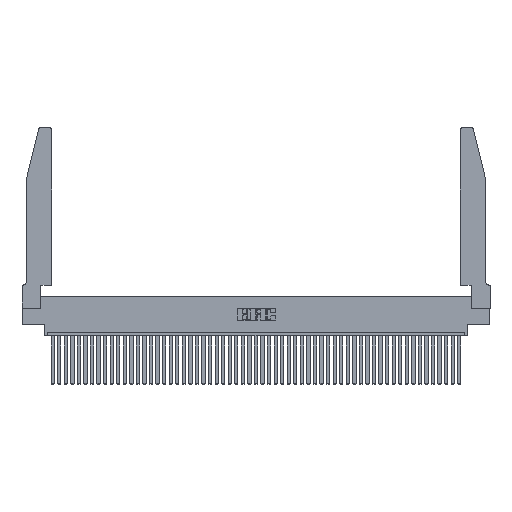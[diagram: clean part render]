
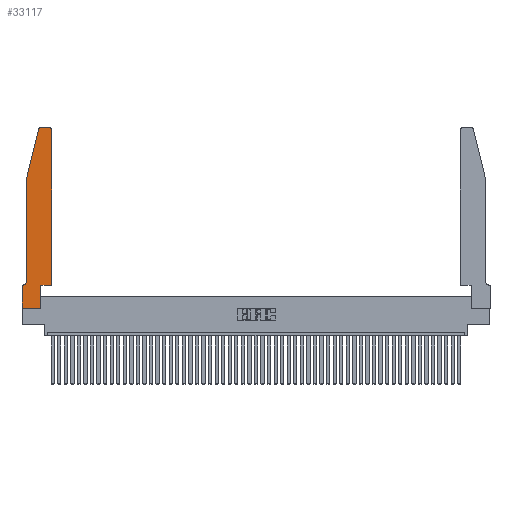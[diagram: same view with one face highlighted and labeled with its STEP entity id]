
A CAD part, top view. The second image highlights one B-rep face of the part: STEP entity #33117.
In plain terms, the highlighted planar face has unit normal (0, 0, 1).
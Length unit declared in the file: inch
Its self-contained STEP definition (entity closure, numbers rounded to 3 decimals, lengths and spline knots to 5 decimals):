
#200 = VECTOR ( 'NONE', #14589, 39.37008 ) ;
#364 = CIRCLE ( 'NONE', #32732, 0.07 ) ;
#743 = EDGE_CURVE ( 'NONE', #23067, #35504, #38774, .T. ) ;
#1401 = VERTEX_POINT ( 'NONE', #21921 ) ;
#3380 = PLANE ( 'NONE',  #35588 ) ;
#3620 = EDGE_CURVE ( 'NONE', #1401, #8414, #23001, .T. ) ;
#3917 = VECTOR ( 'NONE', #47409, 39.37008 ) ;
#4557 = CARTESIAN_POINT ( 'NONE',  ( 0.0055, 0.42, 0.37 ) ) ;
#4806 = CARTESIAN_POINT ( 'NONE',  ( 0.0755, 0.42, 0.37 ) ) ;
#5108 = CARTESIAN_POINT ( 'NONE',  ( 0.284, 2.75, 0.37 ) ) ;
#5520 = EDGE_CURVE ( 'NONE', #13405, #23067, #46718, .T. ) ;
#5816 = CARTESIAN_POINT ( 'NONE',  ( 0.0755, 0.35, 0.37 ) ) ;
#5969 = EDGE_CURVE ( 'NONE', #34957, #36948, #16964, .T. ) ;
#6456 = ORIENTED_EDGE ( 'NONE', *, *, #11098, .T. ) ;
#7323 = LINE ( 'NONE', #26712, #200 ) ;
#8024 = VERTEX_POINT ( 'NONE', #4806 ) ;
#8232 = ORIENTED_EDGE ( 'NONE', *, *, #43882, .T. ) ;
#8414 = VERTEX_POINT ( 'NONE', #21046 ) ;
#9020 = LINE ( 'NONE', #21824, #23318 ) ;
#9536 = VECTOR ( 'NONE', #46431, 39.37008 ) ;
#9809 = CARTESIAN_POINT ( 'NONE',  ( 0.4505, 2.72, 0.37 ) ) ;
#10525 = EDGE_CURVE ( 'NONE', #36948, #22888, #38043, .T. ) ;
#10697 = ORIENTED_EDGE ( 'NONE', *, *, #3620, .T. ) ;
#11098 = EDGE_CURVE ( 'NONE', #24712, #37323, #45056, .T. ) ;
#11150 = CARTESIAN_POINT ( 'NONE',  ( 0.4205, 2.72, 0.37 ) ) ;
#11409 = DIRECTION ( 'NONE',  ( 0., 0., 1. ) ) ;
#12108 = DIRECTION ( 'NONE',  ( 0., 0., 1. ) ) ;
#12191 = VECTOR ( 'NONE', #48499, 39.37008 ) ;
#12938 = CARTESIAN_POINT ( 'NONE',  ( 0., 0., 0.37 ) ) ;
#13211 = CARTESIAN_POINT ( 'NONE',  ( 0.4205, 2.75, 0.37 ) ) ;
#13405 = VERTEX_POINT ( 'NONE', #41623 ) ;
#13851 = CARTESIAN_POINT ( 'NONE',  ( 0.2605, 2.75, 0.37 ) ) ;
#14066 = VECTOR ( 'NONE', #29801, 39.37008 ) ;
#14356 = CARTESIAN_POINT ( 'NONE',  ( 0., 0., 0.37 ) ) ;
#14589 = DIRECTION ( 'NONE',  ( 0., 1., 0. ) ) ;
#14818 = FACE_OUTER_BOUND ( 'NONE', #34378, .T. ) ;
#16098 = CARTESIAN_POINT ( 'NONE',  ( 0.284, 2.72, 0.37 ) ) ;
#16238 = ORIENTED_EDGE ( 'NONE', *, *, #25645, .T. ) ;
#16964 = CIRCLE ( 'NONE', #26918, 0.03 ) ;
#18429 = ORIENTED_EDGE ( 'NONE', *, *, #25961, .T. ) ;
#18447 = ORIENTED_EDGE ( 'NONE', *, *, #37245, .T. ) ;
#18881 = VECTOR ( 'NONE', #34330, 39.37008 ) ;
#19453 = EDGE_CURVE ( 'NONE', #8024, #46375, #364, .T. ) ;
#20429 = VECTOR ( 'NONE', #28317, 39.37008 ) ;
#21046 = CARTESIAN_POINT ( 'NONE',  ( 0.0755, 2., 0.37 ) ) ;
#21333 = CARTESIAN_POINT ( 'NONE',  ( 0.0755, 2., 0.37 ) ) ;
#21422 = CIRCLE ( 'NONE', #41818, 0.03 ) ;
#21824 = CARTESIAN_POINT ( 'NONE',  ( 0.0755, 2., 0.37 ) ) ;
#21921 = CARTESIAN_POINT ( 'NONE',  ( 0.25487, 2.72718, 0.37 ) ) ;
#22302 = CARTESIAN_POINT ( 'NONE',  ( 0.4505, 0.35, 0.37 ) ) ;
#22888 = VERTEX_POINT ( 'NONE', #5108 ) ;
#23001 = LINE ( 'NONE', #21333, #3917 ) ;
#23067 = VERTEX_POINT ( 'NONE', #12938 ) ;
#23318 = VECTOR ( 'NONE', #32634, 39.37008 ) ;
#23591 = DIRECTION ( 'NONE',  ( 1., 0., 0. ) ) ;
#24158 = LINE ( 'NONE', #22302, #14066 ) ;
#24712 = VERTEX_POINT ( 'NONE', #40433 ) ;
#24820 = ORIENTED_EDGE ( 'NONE', *, *, #10525, .T. ) ;
#25645 = EDGE_CURVE ( 'NONE', #46375, #13405, #42434, .T. ) ;
#25932 = ORIENTED_EDGE ( 'NONE', *, *, #5520, .T. ) ;
#25961 = EDGE_CURVE ( 'NONE', #8414, #8024, #9020, .T. ) ;
#26516 = CARTESIAN_POINT ( 'NONE',  ( 0.4505, 0.35, 0.37 ) ) ;
#26712 = CARTESIAN_POINT ( 'NONE',  ( 0.2865, 0.35, 0.37 ) ) ;
#26856 = CARTESIAN_POINT ( 'NONE',  ( 0.4505, 0.35, 0.37 ) ) ;
#26918 = AXIS2_PLACEMENT_3D ( 'NONE', #11150, #11409, #38108 ) ;
#27597 = ORIENTED_EDGE ( 'NONE', *, *, #19453, .T. ) ;
#28032 = CARTESIAN_POINT ( 'NONE',  ( 0.2865, 0., 0.37 ) ) ;
#28317 = DIRECTION ( 'NONE',  ( -1., 0., 0. ) ) ;
#28336 = ORIENTED_EDGE ( 'NONE', *, *, #743, .T. ) ;
#28362 = ORIENTED_EDGE ( 'NONE', *, *, #42085, .T. ) ;
#29801 = DIRECTION ( 'NONE',  ( 0., 1., 0. ) ) ;
#30062 = DIRECTION ( 'NONE',  ( 1., 0., 0. ) ) ;
#30289 = VECTOR ( 'NONE', #40540, 39.37008 ) ;
#32634 = DIRECTION ( 'NONE',  ( 0., -1., 0. ) ) ;
#32732 = AXIS2_PLACEMENT_3D ( 'NONE', #4557, #32733, #36911 ) ;
#32733 = DIRECTION ( 'NONE',  ( 0., 0., -1. ) ) ;
#33117 = ADVANCED_FACE ( 'NONE', ( #14818 ), #3380, .T. ) ;
#34330 = DIRECTION ( 'NONE',  ( 1., 0., 0. ) ) ;
#34378 = EDGE_LOOP ( 'NONE', ( #24820, #28362, #10697, #18429, #27597, #16238, #25932, #28336, #18447, #6456, #8232, #37284 ) ) ;
#34957 = VERTEX_POINT ( 'NONE', #9809 ) ;
#35504 = VERTEX_POINT ( 'NONE', #28032 ) ;
#35588 = AXIS2_PLACEMENT_3D ( 'NONE', #44832, #49006, #30062 ) ;
#36911 = DIRECTION ( 'NONE',  ( -1., 0., 0. ) ) ;
#36948 = VERTEX_POINT ( 'NONE', #13211 ) ;
#37245 = EDGE_CURVE ( 'NONE', #35504, #24712, #7323, .T. ) ;
#37284 = ORIENTED_EDGE ( 'NONE', *, *, #5969, .T. ) ;
#37323 = VERTEX_POINT ( 'NONE', #26856 ) ;
#38043 = LINE ( 'NONE', #13851, #30289 ) ;
#38108 = DIRECTION ( 'NONE',  ( 1., 0., 0. ) ) ;
#38774 = LINE ( 'NONE', #42311, #9536 ) ;
#40433 = CARTESIAN_POINT ( 'NONE',  ( 0.2865, 0.35, 0.37 ) ) ;
#40540 = DIRECTION ( 'NONE',  ( -1., 0., 0. ) ) ;
#41623 = CARTESIAN_POINT ( 'NONE',  ( 0., 0.35, 0.37 ) ) ;
#41818 = AXIS2_PLACEMENT_3D ( 'NONE', #16098, #12108, #23591 ) ;
#42085 = EDGE_CURVE ( 'NONE', #22888, #1401, #21422, .T. ) ;
#42311 = CARTESIAN_POINT ( 'NONE',  ( 0., 0., 0.37 ) ) ;
#42434 = LINE ( 'NONE', #5816, #20429 ) ;
#43004 = CARTESIAN_POINT ( 'NONE',  ( 0.0055, 0.35, 0.37 ) ) ;
#43882 = EDGE_CURVE ( 'NONE', #37323, #34957, #24158, .T. ) ;
#44832 = CARTESIAN_POINT ( 'NONE',  ( 0., 0.35, 0.37 ) ) ;
#45056 = LINE ( 'NONE', #26516, #18881 ) ;
#46375 = VERTEX_POINT ( 'NONE', #43004 ) ;
#46431 = DIRECTION ( 'NONE',  ( 1., 0., 0. ) ) ;
#46718 = LINE ( 'NONE', #14356, #12191 ) ;
#47409 = DIRECTION ( 'NONE',  ( -0.239, -0.971, 0. ) ) ;
#48499 = DIRECTION ( 'NONE',  ( 0., -1., 0. ) ) ;
#49006 = DIRECTION ( 'NONE',  ( 0., 0., 1. ) ) ;
